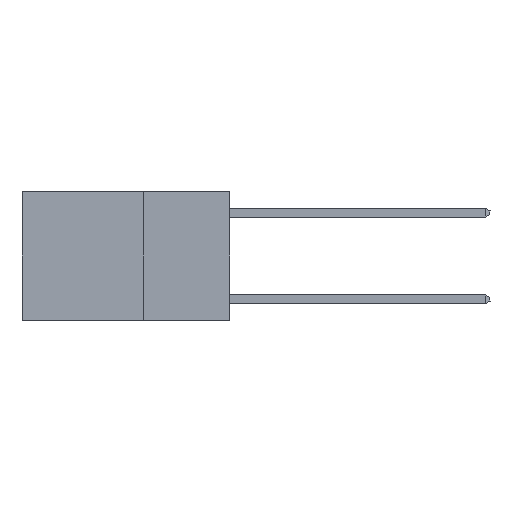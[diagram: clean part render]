
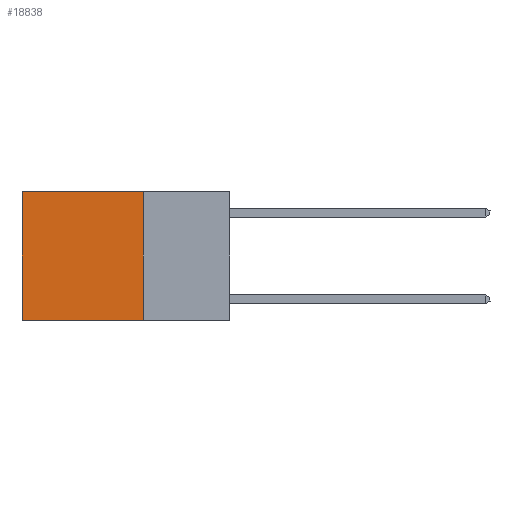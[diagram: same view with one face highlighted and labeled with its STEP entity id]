
A CAD part, left-side view. The second image highlights one B-rep face of the part: STEP entity #18838.
In plain terms, the highlighted planar face has unit normal (-1, 0, 0).
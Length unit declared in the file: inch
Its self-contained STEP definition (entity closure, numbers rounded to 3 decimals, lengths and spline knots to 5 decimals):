
#225 = VERTEX_POINT ( 'NONE', #24916 ) ;
#1092 = EDGE_CURVE ( 'NONE', #11797, #7531, #19791, .T. ) ;
#1115 = ORIENTED_EDGE ( 'NONE', *, *, #24943, .T. ) ;
#4464 = EDGE_CURVE ( 'NONE', #225, #11797, #12634, .T. ) ;
#4816 = ORIENTED_EDGE ( 'NONE', *, *, #4464, .F. ) ;
#5987 = CARTESIAN_POINT ( 'NONE',  ( 0.2625, 0.6, -0.37 ) ) ;
#6535 = VERTEX_POINT ( 'NONE', #30855 ) ;
#7531 = VERTEX_POINT ( 'NONE', #5987 ) ;
#7534 = DIRECTION ( 'NONE',  ( 1., 0., 0. ) ) ;
#7876 = CARTESIAN_POINT ( 'NONE',  ( 0.2625, 0.6, 0. ) ) ;
#8503 = DIRECTION ( 'NONE',  ( 0., 1., 0. ) ) ;
#8656 = DIRECTION ( 'NONE',  ( 0., 0., -1. ) ) ;
#9675 = EDGE_LOOP ( 'NONE', ( #1115, #25210, #4816, #30135 ) ) ;
#10508 = FACE_OUTER_BOUND ( 'NONE', #9675, .T. ) ;
#11797 = VERTEX_POINT ( 'NONE', #24815 ) ;
#12634 = LINE ( 'NONE', #15167, #31028 ) ;
#15167 = CARTESIAN_POINT ( 'NONE',  ( 0.2625, 0.25, 0. ) ) ;
#15278 = VECTOR ( 'NONE', #8503, 39.37008 ) ;
#17149 = PLANE ( 'NONE',  #19755 ) ;
#17262 = VECTOR ( 'NONE', #8656, 39.37008 ) ;
#18838 = ADVANCED_FACE ( 'NONE', ( #10508 ), #17149, .F. ) ;
#19755 = AXIS2_PLACEMENT_3D ( 'NONE', #24403, #7534, #22032 ) ;
#19791 = LINE ( 'NONE', #23918, #24571 ) ;
#19869 = LINE ( 'NONE', #7876, #17262 ) ;
#21540 = DIRECTION ( 'NONE',  ( 0., 1., 0. ) ) ;
#22032 = DIRECTION ( 'NONE',  ( 0., 0., -1. ) ) ;
#23918 = CARTESIAN_POINT ( 'NONE',  ( 0.2625, 0.25, -0.37 ) ) ;
#24403 = CARTESIAN_POINT ( 'NONE',  ( 0.2625, 0.25, 0. ) ) ;
#24571 = VECTOR ( 'NONE', #21540, 39.37008 ) ;
#24815 = CARTESIAN_POINT ( 'NONE',  ( 0.2625, 0.25, -0.37 ) ) ;
#24916 = CARTESIAN_POINT ( 'NONE',  ( 0.2625, 0.25, 0. ) ) ;
#24943 = EDGE_CURVE ( 'NONE', #6535, #7531, #19869, .T. ) ;
#25083 = EDGE_CURVE ( 'NONE', #225, #6535, #27903, .T. ) ;
#25210 = ORIENTED_EDGE ( 'NONE', *, *, #1092, .F. ) ;
#26814 = DIRECTION ( 'NONE',  ( 0., 0., -1. ) ) ;
#27903 = LINE ( 'NONE', #30098, #15278 ) ;
#30098 = CARTESIAN_POINT ( 'NONE',  ( 0.2625, 0.25, 0. ) ) ;
#30135 = ORIENTED_EDGE ( 'NONE', *, *, #25083, .T. ) ;
#30855 = CARTESIAN_POINT ( 'NONE',  ( 0.2625, 0.6, 0. ) ) ;
#31028 = VECTOR ( 'NONE', #26814, 39.37008 ) ;
